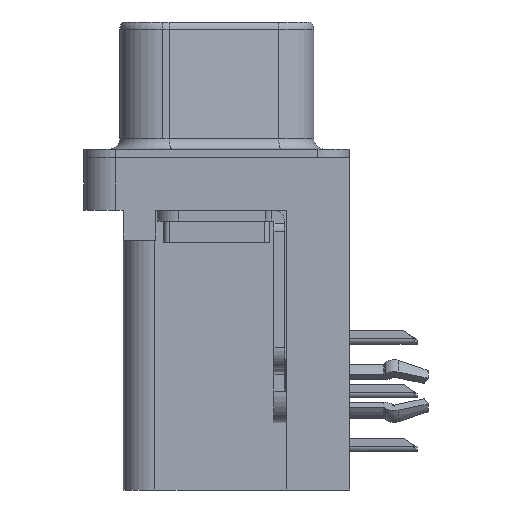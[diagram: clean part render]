
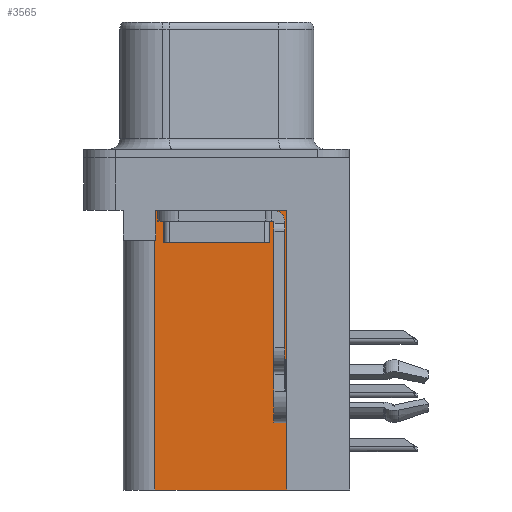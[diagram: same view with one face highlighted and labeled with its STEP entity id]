
A CAD part, left-side view. The second image highlights one B-rep face of the part: STEP entity #3565.
In plain terms, the highlighted planar face has unit normal (-1, 0, 0).
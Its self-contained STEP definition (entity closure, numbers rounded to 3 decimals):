
#458 = ORIENTED_EDGE ( 'NONE', *, *, #25598, .F. ) ;
#570 = EDGE_LOOP ( 'NONE', ( #11230, #19017, #7600, #458, #1406, #7836 ) ) ;
#1406 = ORIENTED_EDGE ( 'NONE', *, *, #13391, .F. ) ;
#1552 = LINE ( 'NONE', #11232, #12769 ) ;
#2745 = VERTEX_POINT ( 'NONE', #21052 ) ;
#2816 = LINE ( 'NONE', #15072, #18063 ) ;
#3147 = DIRECTION ( 'NONE',  ( 0., 1., 0. ) ) ;
#3206 = LINE ( 'NONE', #18329, #24491 ) ;
#3565 = ADVANCED_FACE ( 'NONE', ( #4140 ), #20274, .F. ) ;
#4140 = FACE_OUTER_BOUND ( 'NONE', #570, .T. ) ;
#4396 = CARTESIAN_POINT ( 'NONE',  ( 3.765, 2.925, -15.7 ) ) ;
#4418 = DIRECTION ( 'NONE',  ( 0., 1., 0. ) ) ;
#5969 = LINE ( 'NONE', #4396, #20636 ) ;
#7272 = DIRECTION ( 'NONE',  ( 0., 0., 1. ) ) ;
#7595 = DIRECTION ( 'NONE',  ( 0., 0., -1. ) ) ;
#7600 = ORIENTED_EDGE ( 'NONE', *, *, #25737, .T. ) ;
#7836 = ORIENTED_EDGE ( 'NONE', *, *, #25771, .T. ) ;
#9273 = CARTESIAN_POINT ( 'NONE',  ( 3.765, 2.925, -3.9 ) ) ;
#9906 = VERTEX_POINT ( 'NONE', #9273 ) ;
#10546 = LINE ( 'NONE', #21614, #20616 ) ;
#11203 = VECTOR ( 'NONE', #3147, 1000. ) ;
#11230 = ORIENTED_EDGE ( 'NONE', *, *, #14199, .T. ) ;
#11232 = CARTESIAN_POINT ( 'NONE',  ( 3.765, -3.295, -15.7 ) ) ;
#12769 = VECTOR ( 'NONE', #7272, 1000. ) ;
#13391 = EDGE_CURVE ( 'NONE', #18237, #25168, #3206, .T. ) ;
#14199 = EDGE_CURVE ( 'NONE', #24325, #2745, #16502, .T. ) ;
#15040 = CARTESIAN_POINT ( 'NONE',  ( 3.765, -3.295, -2.5 ) ) ;
#15072 = CARTESIAN_POINT ( 'NONE',  ( 3.765, 0., -3.9 ) ) ;
#15261 = AXIS2_PLACEMENT_3D ( 'NONE', #23706, #20151, #21097 ) ;
#16359 = CARTESIAN_POINT ( 'NONE',  ( 3.765, 2.895, -3.9 ) ) ;
#16502 = LINE ( 'NONE', #15040, #11203 ) ;
#18063 = VECTOR ( 'NONE', #19051, 1000. ) ;
#18123 = CARTESIAN_POINT ( 'NONE',  ( 3.765, -3.295, -2.5 ) ) ;
#18237 = VERTEX_POINT ( 'NONE', #21143 ) ;
#18329 = CARTESIAN_POINT ( 'NONE',  ( 3.765, -3.295, -15.7 ) ) ;
#18713 = CARTESIAN_POINT ( 'NONE',  ( 3.765, 2.925, -15.7 ) ) ;
#19017 = ORIENTED_EDGE ( 'NONE', *, *, #24814, .T. ) ;
#19051 = DIRECTION ( 'NONE',  ( 0., 1., 0. ) ) ;
#20151 = DIRECTION ( 'NONE',  ( 1., 0., 0. ) ) ;
#20274 = PLANE ( 'NONE',  #15261 ) ;
#20616 = VECTOR ( 'NONE', #7595, 1000. ) ;
#20636 = VECTOR ( 'NONE', #22406, 1000. ) ;
#21052 = CARTESIAN_POINT ( 'NONE',  ( 3.765, 2.895, -2.5 ) ) ;
#21097 = DIRECTION ( 'NONE',  ( 0., 0., -1. ) ) ;
#21143 = CARTESIAN_POINT ( 'NONE',  ( 3.765, -3.295, -15.7 ) ) ;
#21614 = CARTESIAN_POINT ( 'NONE',  ( 3.765, 2.895, -3.9 ) ) ;
#22406 = DIRECTION ( 'NONE',  ( 0., 0., 1. ) ) ;
#23706 = CARTESIAN_POINT ( 'NONE',  ( 3.765, -3.295, -15.7 ) ) ;
#24325 = VERTEX_POINT ( 'NONE', #18123 ) ;
#24491 = VECTOR ( 'NONE', #4418, 1000. ) ;
#24814 = EDGE_CURVE ( 'NONE', #2745, #25619, #10546, .T. ) ;
#25168 = VERTEX_POINT ( 'NONE', #18713 ) ;
#25598 = EDGE_CURVE ( 'NONE', #25168, #9906, #5969, .T. ) ;
#25619 = VERTEX_POINT ( 'NONE', #16359 ) ;
#25737 = EDGE_CURVE ( 'NONE', #25619, #9906, #2816, .T. ) ;
#25771 = EDGE_CURVE ( 'NONE', #18237, #24325, #1552, .T. ) ;
